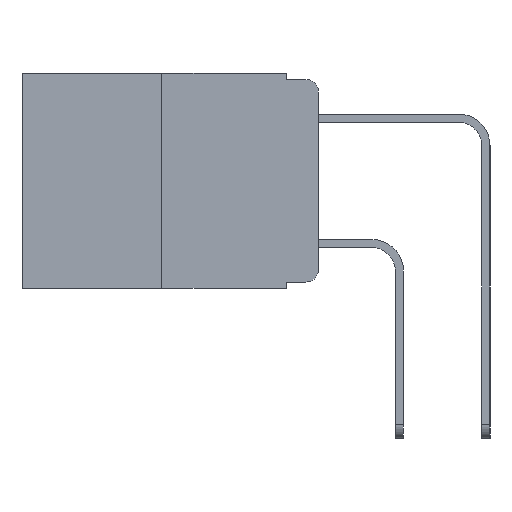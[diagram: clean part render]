
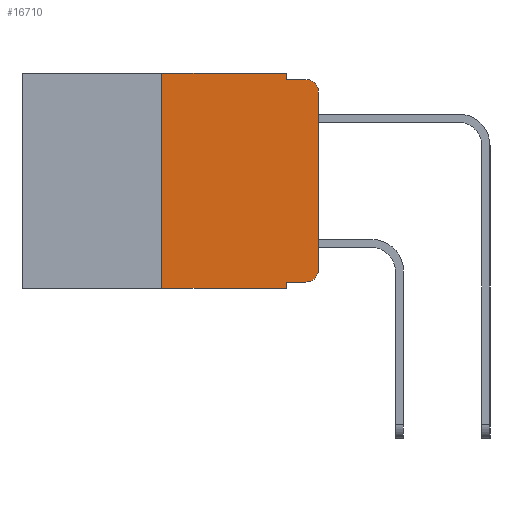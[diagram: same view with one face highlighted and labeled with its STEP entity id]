
A CAD part, left-side view. The second image highlights one B-rep face of the part: STEP entity #16710.
In plain terms, the highlighted planar face has unit normal (-1, 0, 0).
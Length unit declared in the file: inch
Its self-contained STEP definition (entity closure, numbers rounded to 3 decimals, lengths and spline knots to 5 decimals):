
#115 = VECTOR ( 'NONE', #1795, 39.37008 ) ;
#677 = ORIENTED_EDGE ( 'NONE', *, *, #3418, .F. ) ;
#808 = ORIENTED_EDGE ( 'NONE', *, *, #10693, .F. ) ;
#862 = ORIENTED_EDGE ( 'NONE', *, *, #11568, .F. ) ;
#904 = DIRECTION ( 'NONE',  ( 0., 0., -1. ) ) ;
#1256 = VECTOR ( 'NONE', #7580, 39.37008 ) ;
#1462 = LINE ( 'NONE', #16026, #15353 ) ;
#1612 = VERTEX_POINT ( 'NONE', #7411 ) ;
#1795 = DIRECTION ( 'NONE',  ( 0., -1., 0. ) ) ;
#1970 = AXIS2_PLACEMENT_3D ( 'NONE', #1972, #11515, #3391 ) ;
#1972 = CARTESIAN_POINT ( 'NONE',  ( 0., 0.02, -0.03 ) ) ;
#2082 = CARTESIAN_POINT ( 'NONE',  ( 0., 0.051, -0.343 ) ) ;
#2374 = AXIS2_PLACEMENT_3D ( 'NONE', #16957, #9183, #904 ) ;
#3381 = EDGE_CURVE ( 'NONE', #4718, #16646, #13542, .T. ) ;
#3391 = DIRECTION ( 'NONE',  ( 0., 0., -1. ) ) ;
#3410 = CARTESIAN_POINT ( 'NONE',  ( 0., 0.25, 0. ) ) ;
#3418 = EDGE_CURVE ( 'NONE', #8418, #3459, #16611, .T. ) ;
#3451 = ORIENTED_EDGE ( 'NONE', *, *, #7071, .F. ) ;
#3459 = VERTEX_POINT ( 'NONE', #13048 ) ;
#3487 = FACE_OUTER_BOUND ( 'NONE', #13027, .T. ) ;
#3638 = ORIENTED_EDGE ( 'NONE', *, *, #17235, .T. ) ;
#3780 = VECTOR ( 'NONE', #7198, 39.37008 ) ;
#4718 = VERTEX_POINT ( 'NONE', #4750 ) ;
#4750 = CARTESIAN_POINT ( 'NONE',  ( 0., 0.02, -0.333 ) ) ;
#5183 = DIRECTION ( 'NONE',  ( 0., 0., 1. ) ) ;
#5240 = EDGE_CURVE ( 'NONE', #14756, #4718, #14905, .T. ) ;
#6093 = CARTESIAN_POINT ( 'NONE',  ( 0., 0.051, -0.333 ) ) ;
#6271 = CARTESIAN_POINT ( 'NONE',  ( 0., 0.473, 0. ) ) ;
#6347 = VECTOR ( 'NONE', #7499, 39.37008 ) ;
#6816 = ORIENTED_EDGE ( 'NONE', *, *, #12413, .T. ) ;
#7004 = CARTESIAN_POINT ( 'NONE',  ( 0., 0.25, -0.343 ) ) ;
#7071 = EDGE_CURVE ( 'NONE', #14756, #16597, #11006, .T. ) ;
#7132 = ORIENTED_EDGE ( 'NONE', *, *, #3381, .T. ) ;
#7198 = DIRECTION ( 'NONE',  ( 0., 0., -1. ) ) ;
#7325 = ORIENTED_EDGE ( 'NONE', *, *, #15902, .T. ) ;
#7411 = CARTESIAN_POINT ( 'NONE',  ( 0., 0.051, -0.01 ) ) ;
#7499 = DIRECTION ( 'NONE',  ( 0., 0., 1. ) ) ;
#7541 = ORIENTED_EDGE ( 'NONE', *, *, #5240, .T. ) ;
#7580 = DIRECTION ( 'NONE',  ( 0., -1., 0. ) ) ;
#7744 = DIRECTION ( 'NONE',  ( -1., 0., 0. ) ) ;
#7827 = PLANE ( 'NONE',  #2374 ) ;
#7981 = ORIENTED_EDGE ( 'NONE', *, *, #7995, .F. ) ;
#7995 = EDGE_CURVE ( 'NONE', #8797, #8418, #12192, .T. ) ;
#8418 = VERTEX_POINT ( 'NONE', #3410 ) ;
#8797 = VERTEX_POINT ( 'NONE', #7004 ) ;
#9183 = DIRECTION ( 'NONE',  ( 1., 0., 0. ) ) ;
#9256 = VECTOR ( 'NONE', #14069, 39.37008 ) ;
#9801 = VERTEX_POINT ( 'NONE', #12809 ) ;
#9900 = AXIS2_PLACEMENT_3D ( 'NONE', #14241, #7744, #16930 ) ;
#9910 = LINE ( 'NONE', #14063, #6347 ) ;
#10693 = EDGE_CURVE ( 'NONE', #3459, #1612, #1462, .T. ) ;
#11006 = LINE ( 'NONE', #11195, #3780 ) ;
#11069 = CIRCLE ( 'NONE', #1970, 0.02 ) ;
#11195 = CARTESIAN_POINT ( 'NONE',  ( 0., 0.051, 0. ) ) ;
#11515 = DIRECTION ( 'NONE',  ( -1., 0., 0. ) ) ;
#11568 = EDGE_CURVE ( 'NONE', #1612, #9801, #13704, .T. ) ;
#12127 = LINE ( 'NONE', #15497, #1256 ) ;
#12192 = LINE ( 'NONE', #13168, #15631 ) ;
#12413 = EDGE_CURVE ( 'NONE', #13289, #9801, #11069, .T. ) ;
#12796 = CARTESIAN_POINT ( 'NONE',  ( 0., 0.051, -0.333 ) ) ;
#12809 = CARTESIAN_POINT ( 'NONE',  ( 0., 0.02, -0.01 ) ) ;
#13021 = CARTESIAN_POINT ( 'NONE',  ( 0., 0., -0.313 ) ) ;
#13027 = EDGE_LOOP ( 'NONE', ( #7325, #6816, #862, #808, #677, #7981, #3638, #3451, #7541, #7132 ) ) ;
#13048 = CARTESIAN_POINT ( 'NONE',  ( 0., 0.051, 0. ) ) ;
#13168 = CARTESIAN_POINT ( 'NONE',  ( 0., 0.25, 0. ) ) ;
#13289 = VERTEX_POINT ( 'NONE', #16134 ) ;
#13458 = DIRECTION ( 'NONE',  ( 0., 0., -1. ) ) ;
#13542 = CIRCLE ( 'NONE', #9900, 0.02 ) ;
#13704 = LINE ( 'NONE', #15303, #115 ) ;
#14005 = DIRECTION ( 'NONE',  ( 0., -1., 0. ) ) ;
#14063 = CARTESIAN_POINT ( 'NONE',  ( 0., 0., 0. ) ) ;
#14069 = DIRECTION ( 'NONE',  ( 0., -1., 0. ) ) ;
#14241 = CARTESIAN_POINT ( 'NONE',  ( 0., 0.02, -0.313 ) ) ;
#14756 = VERTEX_POINT ( 'NONE', #12796 ) ;
#14905 = LINE ( 'NONE', #6093, #15741 ) ;
#15303 = CARTESIAN_POINT ( 'NONE',  ( 0., 0.051, -0.01 ) ) ;
#15353 = VECTOR ( 'NONE', #13458, 39.37008 ) ;
#15497 = CARTESIAN_POINT ( 'NONE',  ( 0., 0.473, -0.343 ) ) ;
#15631 = VECTOR ( 'NONE', #5183, 39.37008 ) ;
#15741 = VECTOR ( 'NONE', #14005, 39.37008 ) ;
#15902 = EDGE_CURVE ( 'NONE', #16646, #13289, #9910, .T. ) ;
#16026 = CARTESIAN_POINT ( 'NONE',  ( 0., 0.051, 0. ) ) ;
#16134 = CARTESIAN_POINT ( 'NONE',  ( 0., 0., -0.03 ) ) ;
#16597 = VERTEX_POINT ( 'NONE', #2082 ) ;
#16611 = LINE ( 'NONE', #6271, #9256 ) ;
#16646 = VERTEX_POINT ( 'NONE', #13021 ) ;
#16710 = ADVANCED_FACE ( 'NONE', ( #3487 ), #7827, .F. ) ;
#16930 = DIRECTION ( 'NONE',  ( 0., 0., -1. ) ) ;
#16957 = CARTESIAN_POINT ( 'NONE',  ( 0., 0.473, 0. ) ) ;
#17235 = EDGE_CURVE ( 'NONE', #8797, #16597, #12127, .T. ) ;
